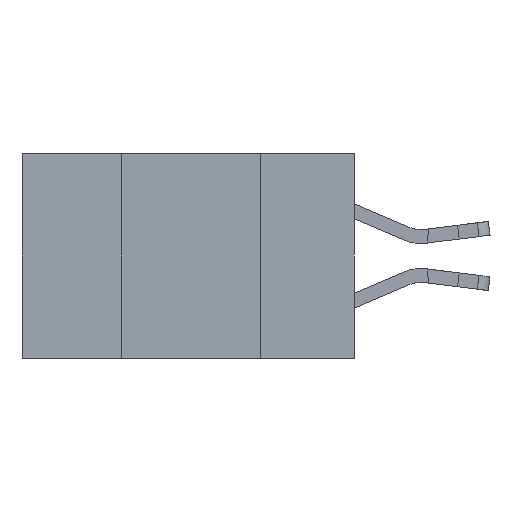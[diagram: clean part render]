
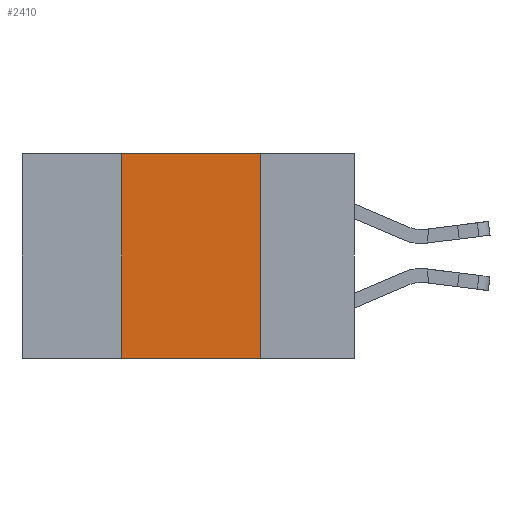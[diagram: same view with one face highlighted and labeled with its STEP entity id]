
A CAD part, left-side view. The second image highlights one B-rep face of the part: STEP entity #2410.
In plain terms, the highlighted planar face has unit normal (-1, 0, 0).
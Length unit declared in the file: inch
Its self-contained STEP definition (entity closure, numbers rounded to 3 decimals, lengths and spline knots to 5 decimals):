
#637 = CARTESIAN_POINT ( 'NONE',  ( 0., 0.42, -0.37 ) ) ;
#1012 = CARTESIAN_POINT ( 'NONE',  ( 0., 0.6, 0. ) ) ;
#1977 = LINE ( 'NONE', #1012, #3053 ) ;
#2410 = ADVANCED_FACE ( 'NONE', ( #10333 ), #5693, .F. ) ;
#2506 = CARTESIAN_POINT ( 'NONE',  ( 0., 0.17, 0. ) ) ;
#2677 = EDGE_CURVE ( 'NONE', #8416, #7904, #4524, .T. ) ;
#2827 = LINE ( 'NONE', #637, #3381 ) ;
#3053 = VECTOR ( 'NONE', #9293, 39.37008 ) ;
#3071 = ORIENTED_EDGE ( 'NONE', *, *, #6709, .T. ) ;
#3181 = ORIENTED_EDGE ( 'NONE', *, *, #5923, .F. ) ;
#3381 = VECTOR ( 'NONE', #6080, 39.37008 ) ;
#3589 = LINE ( 'NONE', #9292, #8422 ) ;
#3710 = CARTESIAN_POINT ( 'NONE',  ( 0., 0.17, -0.37 ) ) ;
#3881 = DIRECTION ( 'NONE',  ( 1., 0., 0. ) ) ;
#4491 = ORIENTED_EDGE ( 'NONE', *, *, #2677, .F. ) ;
#4524 = LINE ( 'NONE', #3710, #10534 ) ;
#5693 = PLANE ( 'NONE',  #6408 ) ;
#5923 = EDGE_CURVE ( 'NONE', #6299, #9966, #2827, .T. ) ;
#6080 = DIRECTION ( 'NONE',  ( 0., 0., 1. ) ) ;
#6134 = ORIENTED_EDGE ( 'NONE', *, *, #8022, .F. ) ;
#6161 = DIRECTION ( 'NONE',  ( 0., 0., -1. ) ) ;
#6299 = VERTEX_POINT ( 'NONE', #6903 ) ;
#6408 = AXIS2_PLACEMENT_3D ( 'NONE', #8713, #3881, #8825 ) ;
#6672 = DIRECTION ( 'NONE',  ( 0., -1., 0. ) ) ;
#6709 = EDGE_CURVE ( 'NONE', #6299, #7904, #3589, .T. ) ;
#6903 = CARTESIAN_POINT ( 'NONE',  ( 0., 0.42, -0.37 ) ) ;
#7317 = CARTESIAN_POINT ( 'NONE',  ( 0., 0.17, -0.37 ) ) ;
#7904 = VERTEX_POINT ( 'NONE', #7317 ) ;
#8022 = EDGE_CURVE ( 'NONE', #9966, #8416, #1977, .T. ) ;
#8416 = VERTEX_POINT ( 'NONE', #2506 ) ;
#8422 = VECTOR ( 'NONE', #6672, 39.37008 ) ;
#8713 = CARTESIAN_POINT ( 'NONE',  ( 0., 0.6, 0. ) ) ;
#8825 = DIRECTION ( 'NONE',  ( 0., 0., -1. ) ) ;
#9292 = CARTESIAN_POINT ( 'NONE',  ( 0., 0.6, -0.37 ) ) ;
#9293 = DIRECTION ( 'NONE',  ( 0., -1., 0. ) ) ;
#9753 = EDGE_LOOP ( 'NONE', ( #4491, #6134, #3181, #3071 ) ) ;
#9966 = VERTEX_POINT ( 'NONE', #10242 ) ;
#10242 = CARTESIAN_POINT ( 'NONE',  ( 0., 0.42, 0. ) ) ;
#10333 = FACE_OUTER_BOUND ( 'NONE', #9753, .T. ) ;
#10534 = VECTOR ( 'NONE', #6161, 39.37008 ) ;
